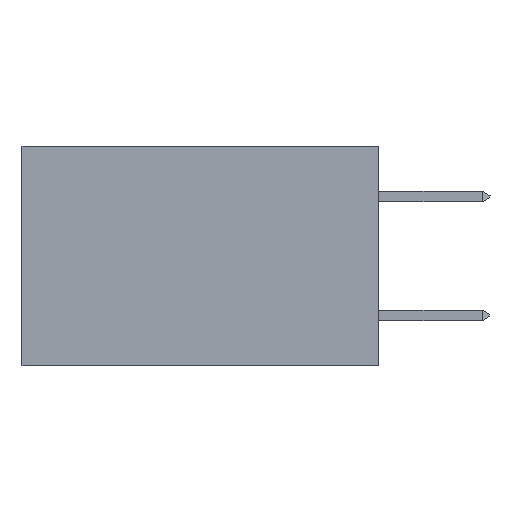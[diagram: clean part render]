
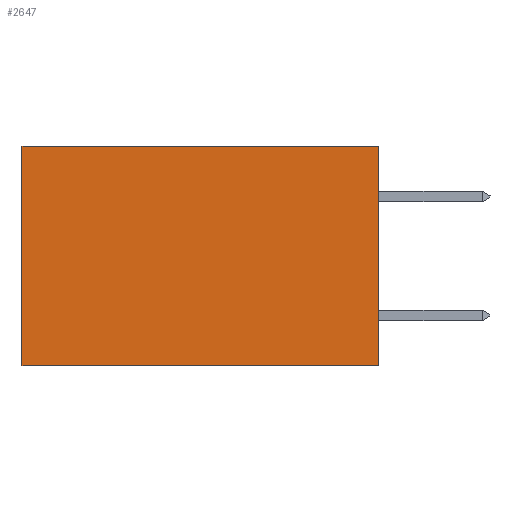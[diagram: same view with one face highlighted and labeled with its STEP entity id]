
A CAD part, left-side view. The second image highlights one B-rep face of the part: STEP entity #2647.
In plain terms, the highlighted planar face has unit normal (-1, 0, 0).
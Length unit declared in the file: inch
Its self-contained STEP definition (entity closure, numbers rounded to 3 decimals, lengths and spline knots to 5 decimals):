
#1118 = CARTESIAN_POINT ( 'NONE',  ( 0.2615, 0., -0.37 ) ) ;
#1206 = CARTESIAN_POINT ( 'NONE',  ( 0.2615, 0.6, -0.37 ) ) ;
#2009 = FACE_OUTER_BOUND ( 'NONE', #16471, .T. ) ;
#2647 = ADVANCED_FACE ( 'NONE', ( #2009 ), #10275, .F. ) ;
#2771 = DIRECTION ( 'NONE',  ( 0., 1., 0. ) ) ;
#3289 = DIRECTION ( 'NONE',  ( 0., 0., -1. ) ) ;
#5223 = VECTOR ( 'NONE', #13574, 39.37008 ) ;
#5402 = EDGE_CURVE ( 'NONE', #7803, #6318, #9214, .T. ) ;
#5439 = EDGE_CURVE ( 'NONE', #7803, #17042, #15269, .T. ) ;
#5567 = CARTESIAN_POINT ( 'NONE',  ( 0.2615, 0., 0. ) ) ;
#5614 = DIRECTION ( 'NONE',  ( 0., 0., -1. ) ) ;
#6318 = VERTEX_POINT ( 'NONE', #17613 ) ;
#6332 = ORIENTED_EDGE ( 'NONE', *, *, #5402, .T. ) ;
#6882 = VECTOR ( 'NONE', #2771, 39.37008 ) ;
#7803 = VERTEX_POINT ( 'NONE', #5567 ) ;
#7899 = CARTESIAN_POINT ( 'NONE',  ( 0.2615, 0., -0.37 ) ) ;
#8933 = EDGE_CURVE ( 'NONE', #6318, #13805, #15345, .T. ) ;
#8992 = DIRECTION ( 'NONE',  ( 1., 0., 0. ) ) ;
#9214 = LINE ( 'NONE', #14808, #6882 ) ;
#9478 = DIRECTION ( 'NONE',  ( 0., 0., -1. ) ) ;
#10275 = PLANE ( 'NONE',  #15908 ) ;
#10320 = ORIENTED_EDGE ( 'NONE', *, *, #10762, .F. ) ;
#10762 = EDGE_CURVE ( 'NONE', #17042, #13805, #17637, .T. ) ;
#11122 = ORIENTED_EDGE ( 'NONE', *, *, #5439, .F. ) ;
#12872 = CARTESIAN_POINT ( 'NONE',  ( 0.2615, 0., -0.37 ) ) ;
#13574 = DIRECTION ( 'NONE',  ( 0., 1., 0. ) ) ;
#13805 = VERTEX_POINT ( 'NONE', #16271 ) ;
#14808 = CARTESIAN_POINT ( 'NONE',  ( 0.2615, 0., 0. ) ) ;
#15179 = VECTOR ( 'NONE', #5614, 39.37008 ) ;
#15269 = LINE ( 'NONE', #1118, #15179 ) ;
#15345 = LINE ( 'NONE', #1206, #17794 ) ;
#15878 = CARTESIAN_POINT ( 'NONE',  ( 0.2615, 0., -0.37 ) ) ;
#15908 = AXIS2_PLACEMENT_3D ( 'NONE', #15878, #8992, #3289 ) ;
#16271 = CARTESIAN_POINT ( 'NONE',  ( 0.2615, 0.6, -0.37 ) ) ;
#16471 = EDGE_LOOP ( 'NONE', ( #16524, #10320, #11122, #6332 ) ) ;
#16524 = ORIENTED_EDGE ( 'NONE', *, *, #8933, .T. ) ;
#17042 = VERTEX_POINT ( 'NONE', #12872 ) ;
#17613 = CARTESIAN_POINT ( 'NONE',  ( 0.2615, 0.6, 0. ) ) ;
#17637 = LINE ( 'NONE', #7899, #5223 ) ;
#17794 = VECTOR ( 'NONE', #9478, 39.37008 ) ;
